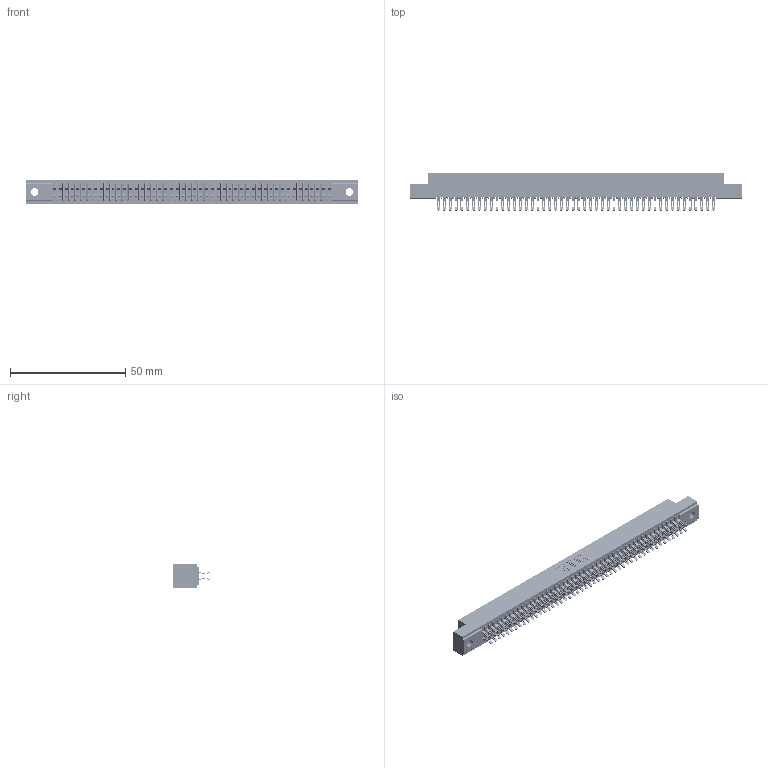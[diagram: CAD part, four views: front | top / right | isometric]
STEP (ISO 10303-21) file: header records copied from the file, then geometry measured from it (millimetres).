
FILE_DESCRIPTION (( 'STEP AP203' ), '1' );
FILE_NAME ('391-096-555-202.STEP', '2018-08-09T18:44:11', ( '' ), ( '' ), 'SwSTEP 2.0', 'SolidWorks 2016', '' );
FILE_SCHEMA (( 'CONFIG_CONTROL_DESIGN' ));
Length unit declared in the file: inch
Products named in the file (3): 341 Part_.128 (3.25) Dia Mounting Holes; 341-292-001_341-292-155; 391-096-555-202
Assembly tree (97 placements, depth 2):
  391-096-555-202
    341 Part_.128 (3.25) Dia Mounting Holes
    341-292-001_341-292-155  x96
Bounding box: 144.15 x 16.31 x 10.16 mm (x, y, z)
Volume: 10731.6 mm3; surface area: 19771.9 mm2
Topology: 97 solids, 97 shells, 7604 faces, 22732 edges, 14798 vertices
Faces by surface type: plane 4100, cylinder 3312, sphere 98, torus 94
Entity records: 57763 total; most frequent: CARTESIAN_POINT 9618, ORIENTED_EDGE 9548, DIRECTION 9320, EDGE_CURVE 4774, LINE 3848, VECTOR 3848, VERTEX_POINT 3018, AXIS2_PLACEMENT_3D 2736
